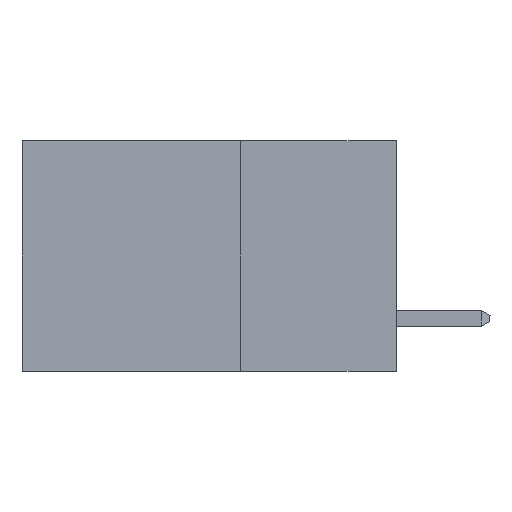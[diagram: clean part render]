
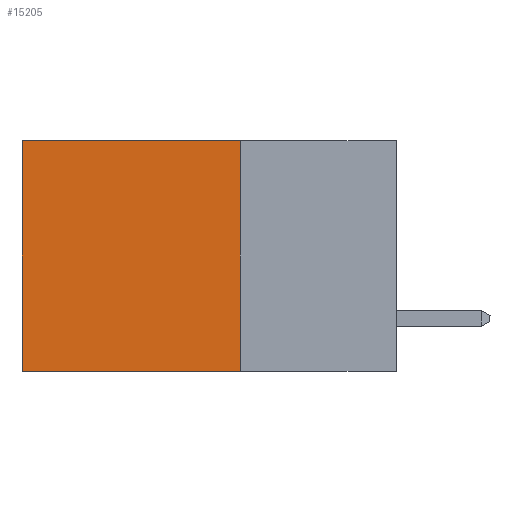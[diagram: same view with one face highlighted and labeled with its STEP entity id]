
A CAD part, left-side view. The second image highlights one B-rep face of the part: STEP entity #15205.
In plain terms, the highlighted planar face has unit normal (-1, 0, 0).
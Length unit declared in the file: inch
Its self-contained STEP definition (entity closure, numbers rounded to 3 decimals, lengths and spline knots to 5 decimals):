
#184 = DIRECTION ( 'NONE',  ( 0., 0., -1. ) ) ;
#859 = EDGE_CURVE ( 'NONE', #18405, #18749, #2790, .T. ) ;
#2171 = EDGE_CURVE ( 'NONE', #18749, #20674, #3893, .T. ) ;
#2275 = LINE ( 'NONE', #8137, #18842 ) ;
#2790 = LINE ( 'NONE', #15466, #7859 ) ;
#3893 = LINE ( 'NONE', #12968, #14218 ) ;
#4304 = AXIS2_PLACEMENT_3D ( 'NONE', #12986, #11500, #184 ) ;
#4606 = CARTESIAN_POINT ( 'NONE',  ( 0.298, 0.6, 0. ) ) ;
#6393 = DIRECTION ( 'NONE',  ( 0., 0., -1. ) ) ;
#6904 = ORIENTED_EDGE ( 'NONE', *, *, #16567, .F. ) ;
#7859 = VECTOR ( 'NONE', #16764, 39.37008 ) ;
#8137 = CARTESIAN_POINT ( 'NONE',  ( 0.298, 0.25, -0.37 ) ) ;
#8335 = PLANE ( 'NONE',  #4304 ) ;
#9450 = CARTESIAN_POINT ( 'NONE',  ( 0.298, 0.6, -0.37 ) ) ;
#10563 = VECTOR ( 'NONE', #6393, 39.37008 ) ;
#11062 = LINE ( 'NONE', #11331, #10563 ) ;
#11311 = ORIENTED_EDGE ( 'NONE', *, *, #18322, .F. ) ;
#11331 = CARTESIAN_POINT ( 'NONE',  ( 0.298, 0.25, 0. ) ) ;
#11500 = DIRECTION ( 'NONE',  ( 1., 0., 0. ) ) ;
#12300 = VERTEX_POINT ( 'NONE', #19584 ) ;
#12968 = CARTESIAN_POINT ( 'NONE',  ( 0.298, 0.6, 0. ) ) ;
#12986 = CARTESIAN_POINT ( 'NONE',  ( 0.298, 0.25, 0. ) ) ;
#13510 = EDGE_LOOP ( 'NONE', ( #18001, #11311, #6904, #18525 ) ) ;
#14218 = VECTOR ( 'NONE', #19369, 39.37008 ) ;
#15205 = ADVANCED_FACE ( 'NONE', ( #15382 ), #8335, .F. ) ;
#15382 = FACE_OUTER_BOUND ( 'NONE', #13510, .T. ) ;
#15466 = CARTESIAN_POINT ( 'NONE',  ( 0.298, 0.25, 0. ) ) ;
#16567 = EDGE_CURVE ( 'NONE', #18405, #12300, #11062, .T. ) ;
#16764 = DIRECTION ( 'NONE',  ( 0., 1., 0. ) ) ;
#17871 = CARTESIAN_POINT ( 'NONE',  ( 0.298, 0.25, 0. ) ) ;
#18001 = ORIENTED_EDGE ( 'NONE', *, *, #2171, .T. ) ;
#18322 = EDGE_CURVE ( 'NONE', #12300, #20674, #2275, .T. ) ;
#18405 = VERTEX_POINT ( 'NONE', #17871 ) ;
#18525 = ORIENTED_EDGE ( 'NONE', *, *, #859, .T. ) ;
#18749 = VERTEX_POINT ( 'NONE', #4606 ) ;
#18842 = VECTOR ( 'NONE', #19468, 39.37008 ) ;
#19369 = DIRECTION ( 'NONE',  ( 0., 0., -1. ) ) ;
#19468 = DIRECTION ( 'NONE',  ( 0., 1., 0. ) ) ;
#19584 = CARTESIAN_POINT ( 'NONE',  ( 0.298, 0.25, -0.37 ) ) ;
#20674 = VERTEX_POINT ( 'NONE', #9450 ) ;
